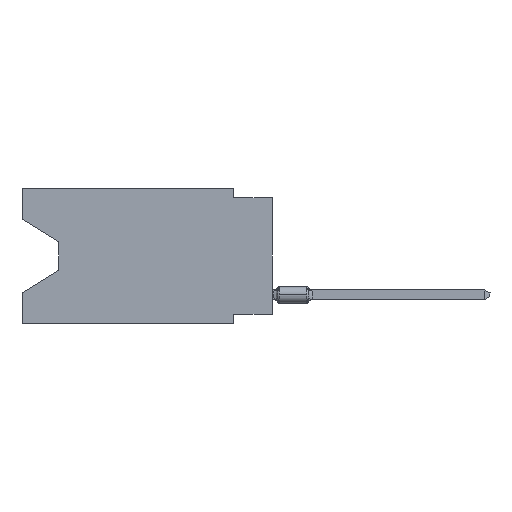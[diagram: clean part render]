
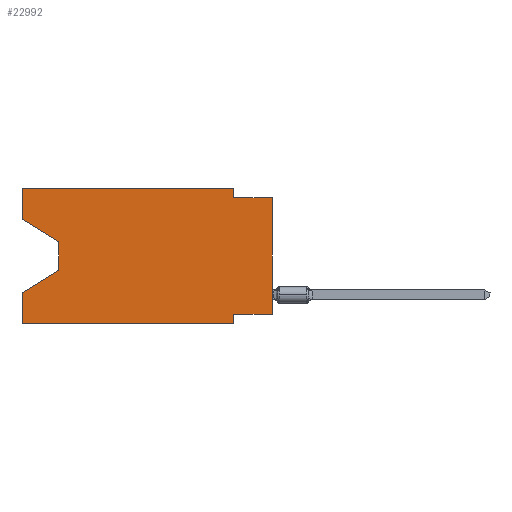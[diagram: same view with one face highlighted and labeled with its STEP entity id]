
A CAD part, left-side view. The second image highlights one B-rep face of the part: STEP entity #22992.
In plain terms, the highlighted planar face has unit normal (-1, 0, 0).
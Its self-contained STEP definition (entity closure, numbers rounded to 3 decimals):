
#43 = VERTEX_POINT ( 'NONE', #15886 ) ;
#195 = CARTESIAN_POINT ( 'NONE',  ( 0., 16.383, 0. ) ) ;
#1978 = ORIENTED_EDGE ( 'NONE', *, *, #22735, .F. ) ;
#3063 = DIRECTION ( 'NONE',  ( 0., 0.855, -0.519 ) ) ;
#3513 = CARTESIAN_POINT ( 'NONE',  ( 0., 0., -8.255 ) ) ;
#3833 = CARTESIAN_POINT ( 'NONE',  ( 0., 16.383, 0. ) ) ;
#5118 = CARTESIAN_POINT ( 'NONE',  ( 0., 16.383, 0. ) ) ;
#5778 = ORIENTED_EDGE ( 'NONE', *, *, #32362, .T. ) ;
#5905 = LINE ( 'NONE', #10761, #46738 ) ;
#6194 = CARTESIAN_POINT ( 'NONE',  ( 0., 16.383, -2.038 ) ) ;
#6709 = DIRECTION ( 'NONE',  ( 0., 0., -1. ) ) ;
#7145 = EDGE_CURVE ( 'NONE', #38985, #29833, #5905, .T. ) ;
#8809 = CARTESIAN_POINT ( 'NONE',  ( 0., 13.97, -5.385 ) ) ;
#10761 = CARTESIAN_POINT ( 'NONE',  ( 0., 16.383, -8.89 ) ) ;
#11574 = CARTESIAN_POINT ( 'NONE',  ( 0., 0., -0.635 ) ) ;
#11617 = VECTOR ( 'NONE', #43542, 1000. ) ;
#12717 = LINE ( 'NONE', #46551, #28270 ) ;
#13338 = VERTEX_POINT ( 'NONE', #44297 ) ;
#14960 = ORIENTED_EDGE ( 'NONE', *, *, #18165, .T. ) ;
#15481 = LINE ( 'NONE', #5118, #11617 ) ;
#15843 = CARTESIAN_POINT ( 'NONE',  ( 0., 16.383, -8.89 ) ) ;
#15886 = CARTESIAN_POINT ( 'NONE',  ( 0., 0., -0.635 ) ) ;
#15943 = LINE ( 'NONE', #6194, #52996 ) ;
#16159 = LINE ( 'NONE', #38451, #36160 ) ;
#16927 = DIRECTION ( 'NONE',  ( 0., 1., 0. ) ) ;
#18165 = EDGE_CURVE ( 'NONE', #57584, #25438, #49721, .T. ) ;
#18399 = VECTOR ( 'NONE', #3063, 1000. ) ;
#18646 = ORIENTED_EDGE ( 'NONE', *, *, #48277, .T. ) ;
#18989 = VERTEX_POINT ( 'NONE', #3833 ) ;
#19450 = LINE ( 'NONE', #50882, #36141 ) ;
#20073 = CARTESIAN_POINT ( 'NONE',  ( 0., 16.383, -6.852 ) ) ;
#20235 = DIRECTION ( 'NONE',  ( 0., -0.855, -0.519 ) ) ;
#20236 = AXIS2_PLACEMENT_3D ( 'NONE', #48288, #43727, #43116 ) ;
#21346 = CARTESIAN_POINT ( 'NONE',  ( 0., 16.383, 0. ) ) ;
#21665 = CARTESIAN_POINT ( 'NONE',  ( 0., 2.54, -0.635 ) ) ;
#22735 = EDGE_CURVE ( 'NONE', #58904, #56465, #35829, .T. ) ;
#22881 = VECTOR ( 'NONE', #34600, 1000. ) ;
#22992 = ADVANCED_FACE ( 'NONE', ( #28193 ), #25418, .F. ) ;
#23395 = VECTOR ( 'NONE', #55091, 1000. ) ;
#24484 = EDGE_CURVE ( 'NONE', #38985, #25438, #27356, .T. ) ;
#24497 = EDGE_CURVE ( 'NONE', #46156, #59597, #12717, .T. ) ;
#24752 = ORIENTED_EDGE ( 'NONE', *, *, #24497, .F. ) ;
#24993 = EDGE_CURVE ( 'NONE', #56465, #29833, #16159, .T. ) ;
#25155 = LINE ( 'NONE', #52902, #22881 ) ;
#25175 = EDGE_CURVE ( 'NONE', #18989, #46156, #36276, .T. ) ;
#25418 = PLANE ( 'NONE',  #20236 ) ;
#25438 = VERTEX_POINT ( 'NONE', #20073 ) ;
#25552 = VERTEX_POINT ( 'NONE', #34694 ) ;
#26820 = DIRECTION ( 'NONE',  ( 0., -1., 0. ) ) ;
#26833 = CARTESIAN_POINT ( 'NONE',  ( 0., 13.97, -5.385 ) ) ;
#27356 = LINE ( 'NONE', #195, #23395 ) ;
#28193 = FACE_OUTER_BOUND ( 'NONE', #49377, .T. ) ;
#28257 = EDGE_CURVE ( 'NONE', #13338, #57584, #25155, .T. ) ;
#28270 = VECTOR ( 'NONE', #31325, 1000. ) ;
#28551 = ORIENTED_EDGE ( 'NONE', *, *, #36752, .F. ) ;
#29042 = EDGE_CURVE ( 'NONE', #59597, #43, #48491, .T. ) ;
#29510 = ORIENTED_EDGE ( 'NONE', *, *, #25175, .F. ) ;
#29833 = VERTEX_POINT ( 'NONE', #34685 ) ;
#31325 = DIRECTION ( 'NONE',  ( 0., 0., -1. ) ) ;
#32362 = EDGE_CURVE ( 'NONE', #58904, #43, #19450, .T. ) ;
#33342 = CARTESIAN_POINT ( 'NONE',  ( 0., 2.54, -8.255 ) ) ;
#34600 = DIRECTION ( 'NONE',  ( 0., 0., -1. ) ) ;
#34685 = CARTESIAN_POINT ( 'NONE',  ( 0., 2.54, -8.89 ) ) ;
#34694 = CARTESIAN_POINT ( 'NONE',  ( 0., 16.383, -2.038 ) ) ;
#35829 = LINE ( 'NONE', #3513, #36764 ) ;
#36141 = VECTOR ( 'NONE', #47499, 1000. ) ;
#36160 = VECTOR ( 'NONE', #6709, 1000. ) ;
#36276 = LINE ( 'NONE', #21346, #43991 ) ;
#36752 = EDGE_CURVE ( 'NONE', #25552, #18989, #15481, .T. ) ;
#36764 = VECTOR ( 'NONE', #16927, 1000. ) ;
#38451 = CARTESIAN_POINT ( 'NONE',  ( 0., 2.54, -8.89 ) ) ;
#38985 = VERTEX_POINT ( 'NONE', #15843 ) ;
#39521 = VECTOR ( 'NONE', #43023, 1000. ) ;
#43023 = DIRECTION ( 'NONE',  ( 0., -1., 0. ) ) ;
#43116 = DIRECTION ( 'NONE',  ( 0., 0., -1. ) ) ;
#43461 = ORIENTED_EDGE ( 'NONE', *, *, #28257, .T. ) ;
#43542 = DIRECTION ( 'NONE',  ( 0., 0., 1. ) ) ;
#43727 = DIRECTION ( 'NONE',  ( 1., 0., 0. ) ) ;
#43991 = VECTOR ( 'NONE', #26820, 1000. ) ;
#44297 = CARTESIAN_POINT ( 'NONE',  ( 0., 13.97, -3.505 ) ) ;
#46156 = VERTEX_POINT ( 'NONE', #51146 ) ;
#46551 = CARTESIAN_POINT ( 'NONE',  ( 0., 2.54, 0. ) ) ;
#46738 = VECTOR ( 'NONE', #47972, 1000. ) ;
#47499 = DIRECTION ( 'NONE',  ( 0., 0., 1. ) ) ;
#47972 = DIRECTION ( 'NONE',  ( 0., -1., 0. ) ) ;
#48277 = EDGE_CURVE ( 'NONE', #25552, #13338, #15943, .T. ) ;
#48288 = CARTESIAN_POINT ( 'NONE',  ( 0., 16.383, 0. ) ) ;
#48491 = LINE ( 'NONE', #11574, #39521 ) ;
#48720 = ORIENTED_EDGE ( 'NONE', *, *, #24484, .F. ) ;
#49377 = EDGE_LOOP ( 'NONE', ( #18646, #43461, #14960, #48720, #57992, #57826, #1978, #5778, #50130, #24752, #29510, #28551 ) ) ;
#49721 = LINE ( 'NONE', #26833, #18399 ) ;
#50061 = CARTESIAN_POINT ( 'NONE',  ( 0., 0., -8.255 ) ) ;
#50130 = ORIENTED_EDGE ( 'NONE', *, *, #29042, .F. ) ;
#50882 = CARTESIAN_POINT ( 'NONE',  ( 0., 0., 0. ) ) ;
#51146 = CARTESIAN_POINT ( 'NONE',  ( 0., 2.54, 0. ) ) ;
#52902 = CARTESIAN_POINT ( 'NONE',  ( 0., 13.97, -3.505 ) ) ;
#52996 = VECTOR ( 'NONE', #20235, 1000. ) ;
#55091 = DIRECTION ( 'NONE',  ( 0., 0., 1. ) ) ;
#56465 = VERTEX_POINT ( 'NONE', #33342 ) ;
#57584 = VERTEX_POINT ( 'NONE', #8809 ) ;
#57826 = ORIENTED_EDGE ( 'NONE', *, *, #24993, .F. ) ;
#57992 = ORIENTED_EDGE ( 'NONE', *, *, #7145, .T. ) ;
#58904 = VERTEX_POINT ( 'NONE', #50061 ) ;
#59597 = VERTEX_POINT ( 'NONE', #21665 ) ;
